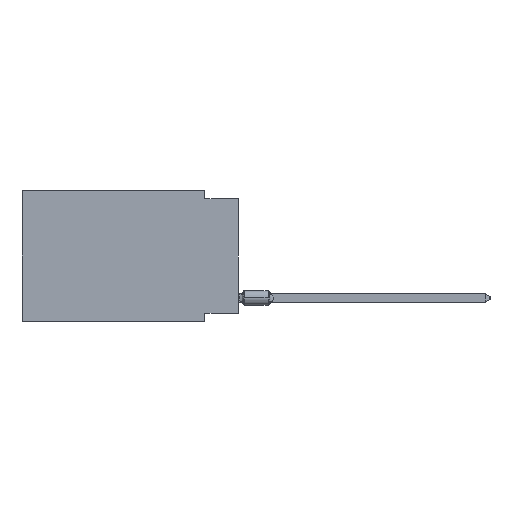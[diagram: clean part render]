
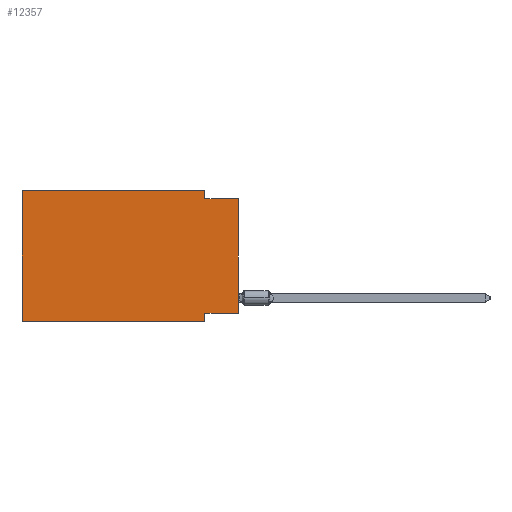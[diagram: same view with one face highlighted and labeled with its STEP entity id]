
A CAD part, left-side view. The second image highlights one B-rep face of the part: STEP entity #12357.
In plain terms, the highlighted planar face has unit normal (-1, 0, 0).
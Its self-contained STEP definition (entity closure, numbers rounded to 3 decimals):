
#1002 = CARTESIAN_POINT ( 'NONE',  ( 0., 16.383, 0. ) ) ;
#1072 = LINE ( 'NONE', #30923, #3034 ) ;
#2150 = EDGE_CURVE ( 'NONE', #48102, #42608, #41756, .T. ) ;
#2545 = EDGE_CURVE ( 'NONE', #43932, #21964, #25301, .T. ) ;
#3034 = VECTOR ( 'NONE', #38989, 1000. ) ;
#3117 = ORIENTED_EDGE ( 'NONE', *, *, #15784, .T. ) ;
#3332 = DIRECTION ( 'NONE',  ( 0., 0., 1. ) ) ;
#3725 = VERTEX_POINT ( 'NONE', #32902 ) ;
#3809 = CARTESIAN_POINT ( 'NONE',  ( 0., 2.54, -9.906 ) ) ;
#4197 = EDGE_CURVE ( 'NONE', #42608, #47362, #34530, .T. ) ;
#5114 = VECTOR ( 'NONE', #20191, 1000. ) ;
#5316 = VECTOR ( 'NONE', #25830, 1000. ) ;
#5984 = EDGE_CURVE ( 'NONE', #48102, #29991, #1072, .T. ) ;
#6266 = CARTESIAN_POINT ( 'NONE',  ( 0., 0., -9.271 ) ) ;
#6830 = PLANE ( 'NONE',  #26029 ) ;
#7322 = FACE_OUTER_BOUND ( 'NONE', #16964, .T. ) ;
#8204 = EDGE_CURVE ( 'NONE', #34440, #29991, #37816, .T. ) ;
#8557 = CARTESIAN_POINT ( 'NONE',  ( 0., 2.54, -9.906 ) ) ;
#10442 = CARTESIAN_POINT ( 'NONE',  ( 0., 16.383, 0. ) ) ;
#11814 = ORIENTED_EDGE ( 'NONE', *, *, #24085, .F. ) ;
#12357 = ADVANCED_FACE ( 'NONE', ( #7322 ), #6830, .F. ) ;
#12390 = ORIENTED_EDGE ( 'NONE', *, *, #17916, .F. ) ;
#14008 = ORIENTED_EDGE ( 'NONE', *, *, #5984, .T. ) ;
#14664 = DIRECTION ( 'NONE',  ( 0., 0., -1. ) ) ;
#15784 = EDGE_CURVE ( 'NONE', #3725, #21964, #18023, .T. ) ;
#16964 = EDGE_LOOP ( 'NONE', ( #3117, #18906, #11814, #27915, #40877, #14008, #36049, #12390 ) ) ;
#17916 = EDGE_CURVE ( 'NONE', #3725, #34440, #47380, .T. ) ;
#18023 = LINE ( 'NONE', #32947, #23966 ) ;
#18906 = ORIENTED_EDGE ( 'NONE', *, *, #2545, .F. ) ;
#18987 = DIRECTION ( 'NONE',  ( 0., 0., -1. ) ) ;
#19242 = CARTESIAN_POINT ( 'NONE',  ( 0., 16.383, 0. ) ) ;
#20191 = DIRECTION ( 'NONE',  ( 0., 0., 1. ) ) ;
#21964 = VERTEX_POINT ( 'NONE', #38649 ) ;
#22044 = CARTESIAN_POINT ( 'NONE',  ( 0., 2.54, 0. ) ) ;
#23966 = VECTOR ( 'NONE', #3332, 1000. ) ;
#24022 = DIRECTION ( 'NONE',  ( 0., 0., -1. ) ) ;
#24085 = EDGE_CURVE ( 'NONE', #47362, #43932, #45600, .T. ) ;
#25301 = LINE ( 'NONE', #38197, #38720 ) ;
#25424 = CARTESIAN_POINT ( 'NONE',  ( 0., 16.383, 0. ) ) ;
#25830 = DIRECTION ( 'NONE',  ( 0., 1., 0. ) ) ;
#26029 = AXIS2_PLACEMENT_3D ( 'NONE', #25424, #26161, #14664 ) ;
#26161 = DIRECTION ( 'NONE',  ( 1., 0., 0. ) ) ;
#27915 = ORIENTED_EDGE ( 'NONE', *, *, #4197, .F. ) ;
#29991 = VERTEX_POINT ( 'NONE', #8557 ) ;
#30858 = DIRECTION ( 'NONE',  ( 0., -1., 0. ) ) ;
#30923 = CARTESIAN_POINT ( 'NONE',  ( 0., 16.383, -9.906 ) ) ;
#32902 = CARTESIAN_POINT ( 'NONE',  ( 0., 0., -9.271 ) ) ;
#32947 = CARTESIAN_POINT ( 'NONE',  ( 0., 0., 0. ) ) ;
#34440 = VERTEX_POINT ( 'NONE', #39774 ) ;
#34530 = LINE ( 'NONE', #1002, #45156 ) ;
#36049 = ORIENTED_EDGE ( 'NONE', *, *, #8204, .F. ) ;
#37040 = DIRECTION ( 'NONE',  ( 0., -1., 0. ) ) ;
#37193 = VECTOR ( 'NONE', #24022, 1000. ) ;
#37816 = LINE ( 'NONE', #3809, #46960 ) ;
#38197 = CARTESIAN_POINT ( 'NONE',  ( 0., 0., -0.635 ) ) ;
#38566 = CARTESIAN_POINT ( 'NONE',  ( 0., 2.54, -0.635 ) ) ;
#38649 = CARTESIAN_POINT ( 'NONE',  ( 0., 0., -0.635 ) ) ;
#38720 = VECTOR ( 'NONE', #37040, 1000. ) ;
#38989 = DIRECTION ( 'NONE',  ( 0., -1., 0. ) ) ;
#39774 = CARTESIAN_POINT ( 'NONE',  ( 0., 2.54, -9.271 ) ) ;
#40877 = ORIENTED_EDGE ( 'NONE', *, *, #2150, .F. ) ;
#41756 = LINE ( 'NONE', #19242, #5114 ) ;
#42608 = VERTEX_POINT ( 'NONE', #10442 ) ;
#42636 = CARTESIAN_POINT ( 'NONE',  ( 0., 2.54, 0. ) ) ;
#43932 = VERTEX_POINT ( 'NONE', #38566 ) ;
#45156 = VECTOR ( 'NONE', #30858, 1000. ) ;
#45600 = LINE ( 'NONE', #42636, #37193 ) ;
#46960 = VECTOR ( 'NONE', #18987, 1000. ) ;
#47008 = CARTESIAN_POINT ( 'NONE',  ( 0., 16.383, -9.906 ) ) ;
#47362 = VERTEX_POINT ( 'NONE', #22044 ) ;
#47380 = LINE ( 'NONE', #6266, #5316 ) ;
#48102 = VERTEX_POINT ( 'NONE', #47008 ) ;
